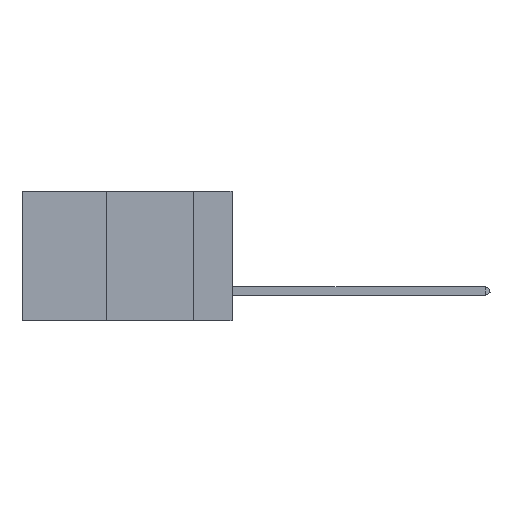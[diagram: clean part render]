
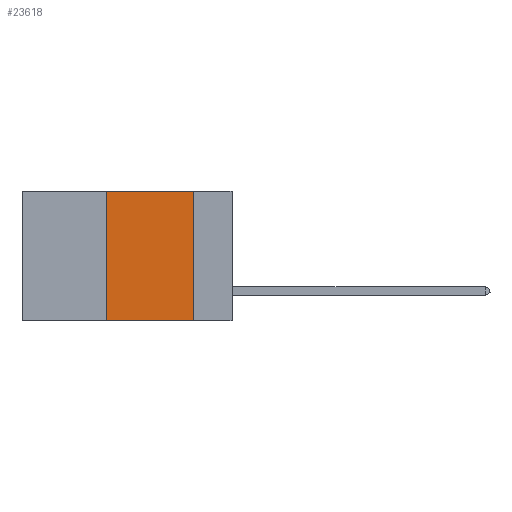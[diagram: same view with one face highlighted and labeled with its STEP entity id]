
A CAD part, left-side view. The second image highlights one B-rep face of the part: STEP entity #23618.
In plain terms, the highlighted planar face has unit normal (-1, 0, 0).
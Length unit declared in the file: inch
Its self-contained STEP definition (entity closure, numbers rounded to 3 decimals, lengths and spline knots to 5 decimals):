
#56 = FACE_OUTER_BOUND ( 'NONE', #19218, .T. ) ;
#173 = EDGE_CURVE ( 'NONE', #24322, #11658, #17179, .T. ) ;
#953 = CARTESIAN_POINT ( 'NONE',  ( 0., 0.11, 0. ) ) ;
#1011 = CARTESIAN_POINT ( 'NONE',  ( 0., 0.36, 0. ) ) ;
#2112 = EDGE_CURVE ( 'NONE', #2866, #4002, #12380, .T. ) ;
#2866 = VERTEX_POINT ( 'NONE', #17573 ) ;
#3296 = CARTESIAN_POINT ( 'NONE',  ( 0., 0.11, -0.37 ) ) ;
#4002 = VERTEX_POINT ( 'NONE', #21144 ) ;
#5834 = CARTESIAN_POINT ( 'NONE',  ( 0., 0.36, -0.37 ) ) ;
#5909 = PLANE ( 'NONE',  #24888 ) ;
#8162 = CARTESIAN_POINT ( 'NONE',  ( 0., 0.6, 0. ) ) ;
#8555 = DIRECTION ( 'NONE',  ( 0., 0., -1. ) ) ;
#10915 = LINE ( 'NONE', #1011, #19585 ) ;
#11155 = ORIENTED_EDGE ( 'NONE', *, *, #2112, .F. ) ;
#11302 = DIRECTION ( 'NONE',  ( 0., -1., 0. ) ) ;
#11402 = VECTOR ( 'NONE', #11302, 39.37008 ) ;
#11426 = CARTESIAN_POINT ( 'NONE',  ( 0., 0.6, -0.37 ) ) ;
#11658 = VERTEX_POINT ( 'NONE', #3296 ) ;
#12380 = LINE ( 'NONE', #8162, #19529 ) ;
#13055 = EDGE_CURVE ( 'NONE', #4002, #11658, #20180, .T. ) ;
#14174 = DIRECTION ( 'NONE',  ( 0., -1., 0. ) ) ;
#14882 = DIRECTION ( 'NONE',  ( 0., 0., 1. ) ) ;
#15981 = DIRECTION ( 'NONE',  ( 1., 0., 0. ) ) ;
#17179 = LINE ( 'NONE', #11426, #11402 ) ;
#17573 = CARTESIAN_POINT ( 'NONE',  ( 0., 0.36, 0. ) ) ;
#19218 = EDGE_LOOP ( 'NONE', ( #20206, #11155, #19537, #19295 ) ) ;
#19295 = ORIENTED_EDGE ( 'NONE', *, *, #173, .T. ) ;
#19529 = VECTOR ( 'NONE', #14174, 39.37008 ) ;
#19537 = ORIENTED_EDGE ( 'NONE', *, *, #21548, .F. ) ;
#19585 = VECTOR ( 'NONE', #14882, 39.37008 ) ;
#19813 = CARTESIAN_POINT ( 'NONE',  ( 0., 0.6, 0. ) ) ;
#20180 = LINE ( 'NONE', #953, #25030 ) ;
#20206 = ORIENTED_EDGE ( 'NONE', *, *, #13055, .F. ) ;
#21144 = CARTESIAN_POINT ( 'NONE',  ( 0., 0.11, 0. ) ) ;
#21548 = EDGE_CURVE ( 'NONE', #24322, #2866, #10915, .T. ) ;
#23378 = DIRECTION ( 'NONE',  ( 0., 0., -1. ) ) ;
#23618 = ADVANCED_FACE ( 'NONE', ( #56 ), #5909, .F. ) ;
#24322 = VERTEX_POINT ( 'NONE', #5834 ) ;
#24888 = AXIS2_PLACEMENT_3D ( 'NONE', #19813, #15981, #23378 ) ;
#25030 = VECTOR ( 'NONE', #8555, 39.37008 ) ;
